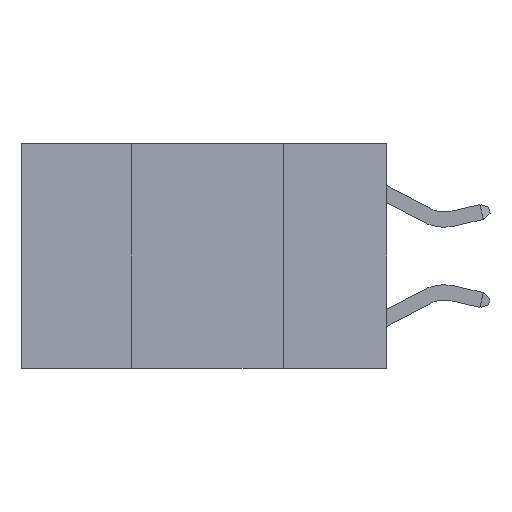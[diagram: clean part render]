
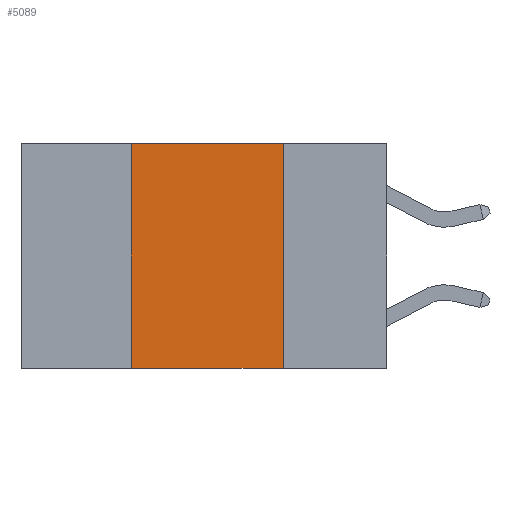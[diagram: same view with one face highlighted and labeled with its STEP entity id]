
A CAD part, left-side view. The second image highlights one B-rep face of the part: STEP entity #5089.
In plain terms, the highlighted planar face has unit normal (-1, 0, 0).
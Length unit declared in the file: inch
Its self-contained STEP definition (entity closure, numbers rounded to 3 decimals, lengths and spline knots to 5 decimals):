
#38 = CARTESIAN_POINT ( 'NONE',  ( 0., 0.17, -0.37 ) ) ;
#55 = DIRECTION ( 'NONE',  ( 0., 0., 1. ) ) ;
#94 = VERTEX_POINT ( 'NONE', #2320 ) ;
#388 = VERTEX_POINT ( 'NONE', #38 ) ;
#585 = LINE ( 'NONE', #9317, #5572 ) ;
#692 = AXIS2_PLACEMENT_3D ( 'NONE', #1399, #10987, #5440 ) ;
#1399 = CARTESIAN_POINT ( 'NONE',  ( 0., 0.6, 0. ) ) ;
#2320 = CARTESIAN_POINT ( 'NONE',  ( 0., 0.17, 0. ) ) ;
#2927 = CARTESIAN_POINT ( 'NONE',  ( 0., 0.42, 0. ) ) ;
#3332 = PLANE ( 'NONE',  #692 ) ;
#3640 = ORIENTED_EDGE ( 'NONE', *, *, #11518, .F. ) ;
#3843 = VECTOR ( 'NONE', #10076, 39.37008 ) ;
#4100 = ORIENTED_EDGE ( 'NONE', *, *, #8876, .F. ) ;
#5089 = ADVANCED_FACE ( 'NONE', ( #7948 ), #3332, .F. ) ;
#5334 = DIRECTION ( 'NONE',  ( 0., 0., -1. ) ) ;
#5440 = DIRECTION ( 'NONE',  ( 0., 0., -1. ) ) ;
#5572 = VECTOR ( 'NONE', #11106, 39.37008 ) ;
#5942 = ORIENTED_EDGE ( 'NONE', *, *, #9503, .F. ) ;
#6011 = VERTEX_POINT ( 'NONE', #11671 ) ;
#6201 = VERTEX_POINT ( 'NONE', #10402 ) ;
#6369 = LINE ( 'NONE', #6399, #8525 ) ;
#6399 = CARTESIAN_POINT ( 'NONE',  ( 0., 0.17, 0. ) ) ;
#6468 = CARTESIAN_POINT ( 'NONE',  ( 0., 0.6, 0. ) ) ;
#6506 = EDGE_LOOP ( 'NONE', ( #4100, #3640, #5942, #11841 ) ) ;
#7196 = LINE ( 'NONE', #6468, #3843 ) ;
#7660 = VECTOR ( 'NONE', #55, 39.37008 ) ;
#7944 = LINE ( 'NONE', #2927, #7660 ) ;
#7948 = FACE_OUTER_BOUND ( 'NONE', #6506, .T. ) ;
#8209 = EDGE_CURVE ( 'NONE', #6011, #388, #585, .T. ) ;
#8525 = VECTOR ( 'NONE', #5334, 39.37008 ) ;
#8876 = EDGE_CURVE ( 'NONE', #94, #388, #6369, .T. ) ;
#9317 = CARTESIAN_POINT ( 'NONE',  ( 0., 0.6, -0.37 ) ) ;
#9503 = EDGE_CURVE ( 'NONE', #6011, #6201, #7944, .T. ) ;
#10076 = DIRECTION ( 'NONE',  ( 0., -1., 0. ) ) ;
#10402 = CARTESIAN_POINT ( 'NONE',  ( 0., 0.42, 0. ) ) ;
#10987 = DIRECTION ( 'NONE',  ( 1., 0., 0. ) ) ;
#11106 = DIRECTION ( 'NONE',  ( 0., -1., 0. ) ) ;
#11518 = EDGE_CURVE ( 'NONE', #6201, #94, #7196, .T. ) ;
#11671 = CARTESIAN_POINT ( 'NONE',  ( 0., 0.42, -0.37 ) ) ;
#11841 = ORIENTED_EDGE ( 'NONE', *, *, #8209, .T. ) ;
